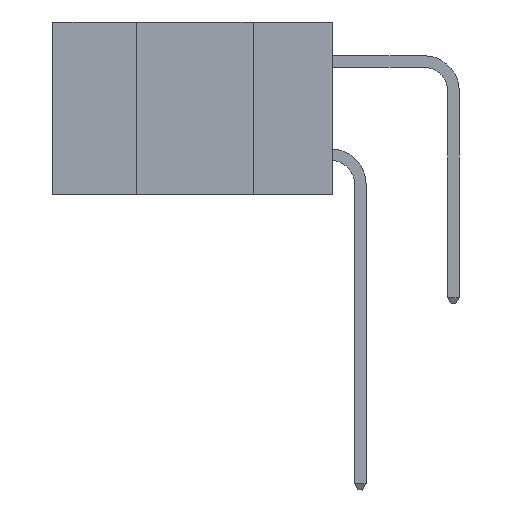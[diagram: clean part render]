
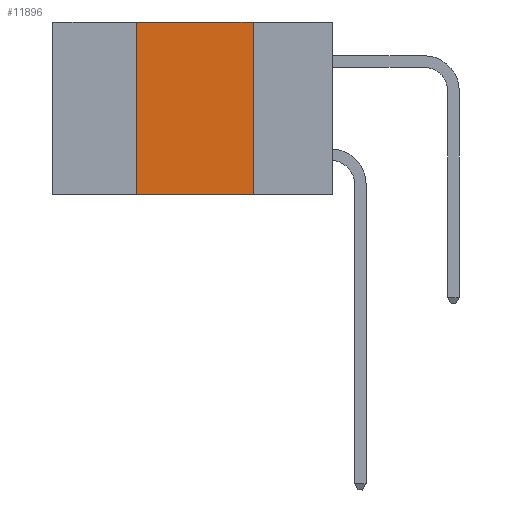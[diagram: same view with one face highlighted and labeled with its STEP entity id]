
A CAD part, left-side view. The second image highlights one B-rep face of the part: STEP entity #11896.
In plain terms, the highlighted planar face has unit normal (-1, 0, 0).
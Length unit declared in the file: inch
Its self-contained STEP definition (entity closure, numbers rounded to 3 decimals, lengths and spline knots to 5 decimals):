
#94 = CARTESIAN_POINT ( 'NONE',  ( 0., 0.17, -0.37 ) ) ;
#120 = ORIENTED_EDGE ( 'NONE', *, *, #12178, .F. ) ;
#161 = DIRECTION ( 'NONE',  ( 0., 0., 1. ) ) ;
#173 = LINE ( 'NONE', #11640, #3726 ) ;
#913 = PLANE ( 'NONE',  #1333 ) ;
#1333 = AXIS2_PLACEMENT_3D ( 'NONE', #5859, #2753, #8674 ) ;
#1671 = CARTESIAN_POINT ( 'NONE',  ( 0., 0.6, -0.37 ) ) ;
#1986 = FACE_OUTER_BOUND ( 'NONE', #3304, .T. ) ;
#2029 = ORIENTED_EDGE ( 'NONE', *, *, #7712, .T. ) ;
#2425 = DIRECTION ( 'NONE',  ( 0., 0., -1. ) ) ;
#2549 = VECTOR ( 'NONE', #161, 39.37008 ) ;
#2753 = DIRECTION ( 'NONE',  ( 1., 0., 0. ) ) ;
#3181 = VERTEX_POINT ( 'NONE', #12436 ) ;
#3304 = EDGE_LOOP ( 'NONE', ( #120, #3481, #3651, #2029 ) ) ;
#3447 = CARTESIAN_POINT ( 'NONE',  ( 0., 0.17, -0.37 ) ) ;
#3481 = ORIENTED_EDGE ( 'NONE', *, *, #4925, .F. ) ;
#3651 = ORIENTED_EDGE ( 'NONE', *, *, #12031, .F. ) ;
#3726 = VECTOR ( 'NONE', #7718, 39.37008 ) ;
#4265 = LINE ( 'NONE', #7128, #2549 ) ;
#4601 = VECTOR ( 'NONE', #9427, 39.37008 ) ;
#4700 = CARTESIAN_POINT ( 'NONE',  ( 0., 0.17, 0. ) ) ;
#4925 = EDGE_CURVE ( 'NONE', #3181, #11050, #173, .T. ) ;
#4946 = VERTEX_POINT ( 'NONE', #5045 ) ;
#5045 = CARTESIAN_POINT ( 'NONE',  ( 0., 0.42, -0.37 ) ) ;
#5859 = CARTESIAN_POINT ( 'NONE',  ( 0., 0.6, 0. ) ) ;
#6350 = LINE ( 'NONE', #3447, #7830 ) ;
#7128 = CARTESIAN_POINT ( 'NONE',  ( 0., 0.42, -0.37 ) ) ;
#7712 = EDGE_CURVE ( 'NONE', #4946, #8702, #12514, .T. ) ;
#7718 = DIRECTION ( 'NONE',  ( 0., -1., 0. ) ) ;
#7830 = VECTOR ( 'NONE', #2425, 39.37008 ) ;
#8674 = DIRECTION ( 'NONE',  ( 0., 0., -1. ) ) ;
#8702 = VERTEX_POINT ( 'NONE', #94 ) ;
#9427 = DIRECTION ( 'NONE',  ( 0., -1., 0. ) ) ;
#11050 = VERTEX_POINT ( 'NONE', #4700 ) ;
#11640 = CARTESIAN_POINT ( 'NONE',  ( 0., 0.6, 0. ) ) ;
#11896 = ADVANCED_FACE ( 'NONE', ( #1986 ), #913, .F. ) ;
#12031 = EDGE_CURVE ( 'NONE', #4946, #3181, #4265, .T. ) ;
#12178 = EDGE_CURVE ( 'NONE', #11050, #8702, #6350, .T. ) ;
#12436 = CARTESIAN_POINT ( 'NONE',  ( 0., 0.42, 0. ) ) ;
#12514 = LINE ( 'NONE', #1671, #4601 ) ;
